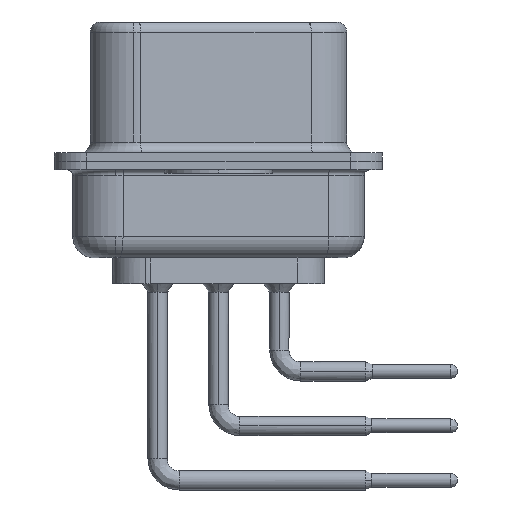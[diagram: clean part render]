
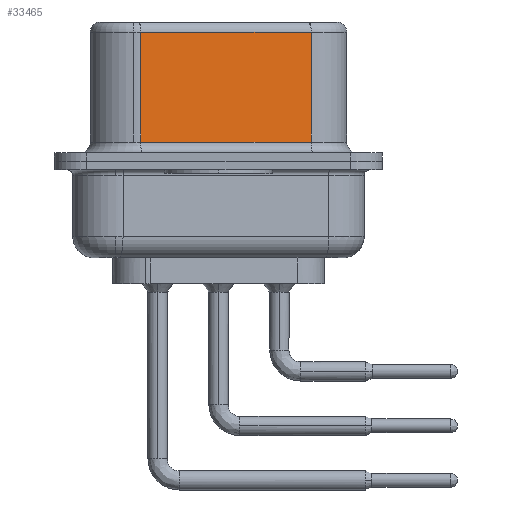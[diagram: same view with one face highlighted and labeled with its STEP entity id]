
A CAD part, left-side view. The second image highlights one B-rep face of the part: STEP entity #33465.
In plain terms, the highlighted planar face has unit normal (-0.985, -0.174, 0).
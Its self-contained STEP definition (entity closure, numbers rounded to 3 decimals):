
#1630 = CARTESIAN_POINT ( 'NONE',  ( 3.73, 3.628, 6.02 ) ) ;
#1634 = VERTEX_POINT ( 'NONE', #16024 ) ;
#2697 = EDGE_CURVE ( 'NONE', #1634, #33003, #24092, .T. ) ;
#4658 = EDGE_LOOP ( 'NONE', ( #18444, #27382, #26414, #28972 ) ) ;
#5501 = LINE ( 'NONE', #25469, #33489 ) ;
#6255 = DIRECTION ( 'NONE',  ( 0.985, 0.174, 0. ) ) ;
#9017 = LINE ( 'NONE', #14812, #34437 ) ;
#9318 = DIRECTION ( 'NONE',  ( 0., 0., -1. ) ) ;
#9607 = DIRECTION ( 'NONE',  ( 0., 0., -1. ) ) ;
#9611 = CARTESIAN_POINT ( 'NONE',  ( 5.132, -4.322, 6.52 ) ) ;
#10185 = CARTESIAN_POINT ( 'NONE',  ( 3.73, 3.628, 0.9 ) ) ;
#10516 = EDGE_CURVE ( 'NONE', #26715, #18154, #5501, .T. ) ;
#14289 = VECTOR ( 'NONE', #34887, 1000. ) ;
#14812 = CARTESIAN_POINT ( 'NONE',  ( 5.132, -4.322, 6.02 ) ) ;
#16024 = CARTESIAN_POINT ( 'NONE',  ( 5.132, -4.322, 6.02 ) ) ;
#17584 = DIRECTION ( 'NONE',  ( -0.174, 0.985, 0. ) ) ;
#18154 = VERTEX_POINT ( 'NONE', #10185 ) ;
#18444 = ORIENTED_EDGE ( 'NONE', *, *, #2697, .F. ) ;
#19267 = EDGE_CURVE ( 'NONE', #1634, #26715, #9017, .T. ) ;
#19542 = PLANE ( 'NONE',  #23156 ) ;
#20264 = CARTESIAN_POINT ( 'NONE',  ( 5.132, -4.322, 0.9 ) ) ;
#21508 = LINE ( 'NONE', #26614, #14289 ) ;
#23156 = AXIS2_PLACEMENT_3D ( 'NONE', #27512, #6255, #25154 ) ;
#24092 = LINE ( 'NONE', #9611, #24941 ) ;
#24941 = VECTOR ( 'NONE', #9607, 1000. ) ;
#25154 = DIRECTION ( 'NONE',  ( -0.174, 0.985, 0. ) ) ;
#25469 = CARTESIAN_POINT ( 'NONE',  ( 3.73, 3.628, 6.52 ) ) ;
#26414 = ORIENTED_EDGE ( 'NONE', *, *, #10516, .T. ) ;
#26614 = CARTESIAN_POINT ( 'NONE',  ( 5.132, -4.322, 0.9 ) ) ;
#26715 = VERTEX_POINT ( 'NONE', #1630 ) ;
#27041 = FACE_OUTER_BOUND ( 'NONE', #4658, .T. ) ;
#27382 = ORIENTED_EDGE ( 'NONE', *, *, #19267, .T. ) ;
#27512 = CARTESIAN_POINT ( 'NONE',  ( 5.132, -4.322, 6.52 ) ) ;
#28972 = ORIENTED_EDGE ( 'NONE', *, *, #34343, .T. ) ;
#33003 = VERTEX_POINT ( 'NONE', #20264 ) ;
#33465 = ADVANCED_FACE ( 'NONE', ( #27041 ), #19542, .F. ) ;
#33489 = VECTOR ( 'NONE', #9318, 1000. ) ;
#34343 = EDGE_CURVE ( 'NONE', #18154, #33003, #21508, .T. ) ;
#34437 = VECTOR ( 'NONE', #17584, 1000. ) ;
#34887 = DIRECTION ( 'NONE',  ( 0.174, -0.985, 0. ) ) ;
